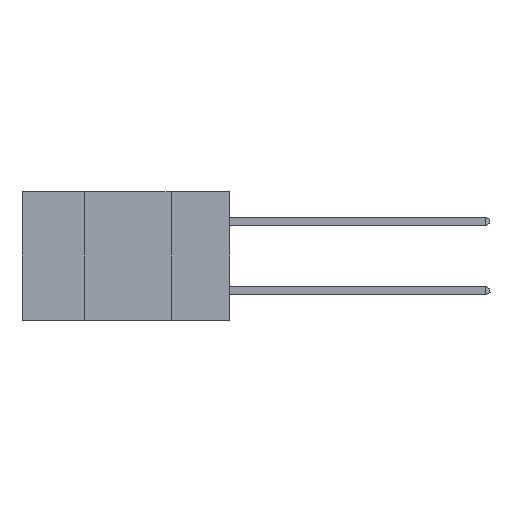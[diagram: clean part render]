
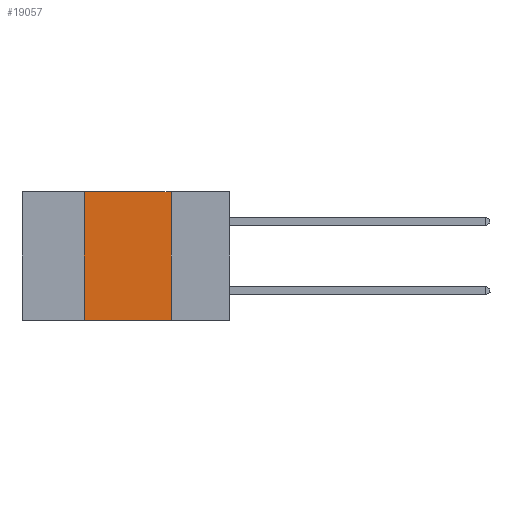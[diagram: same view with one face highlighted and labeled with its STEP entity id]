
A CAD part, left-side view. The second image highlights one B-rep face of the part: STEP entity #19057.
In plain terms, the highlighted planar face has unit normal (-1, 0, 0).
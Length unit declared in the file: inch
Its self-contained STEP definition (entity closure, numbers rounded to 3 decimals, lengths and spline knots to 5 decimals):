
#419 = CARTESIAN_POINT ( 'NONE',  ( 0., 0.17, 0. ) ) ;
#975 = FACE_OUTER_BOUND ( 'NONE', #11754, .T. ) ;
#3410 = EDGE_CURVE ( 'NONE', #18629, #6606, #17385, .T. ) ;
#5823 = VECTOR ( 'NONE', #15433, 39.37008 ) ;
#6005 = CARTESIAN_POINT ( 'NONE',  ( 0., 0.17, 0. ) ) ;
#6018 = PLANE ( 'NONE',  #11530 ) ;
#6328 = VERTEX_POINT ( 'NONE', #6005 ) ;
#6606 = VERTEX_POINT ( 'NONE', #8525 ) ;
#6717 = CARTESIAN_POINT ( 'NONE',  ( 0., 0.42, -0.37 ) ) ;
#6910 = DIRECTION ( 'NONE',  ( 0., 0., -1. ) ) ;
#7424 = ORIENTED_EDGE ( 'NONE', *, *, #16034, .F. ) ;
#8299 = DIRECTION ( 'NONE',  ( 1., 0., 0. ) ) ;
#8525 = CARTESIAN_POINT ( 'NONE',  ( 0., 0.42, 0. ) ) ;
#8859 = CARTESIAN_POINT ( 'NONE',  ( 0., 0.17, -0.37 ) ) ;
#9289 = LINE ( 'NONE', #419, #17434 ) ;
#9847 = CARTESIAN_POINT ( 'NONE',  ( 0., 0.6, -0.37 ) ) ;
#11530 = AXIS2_PLACEMENT_3D ( 'NONE', #21264, #8299, #25635 ) ;
#11754 = EDGE_LOOP ( 'NONE', ( #7424, #23258, #14090, #14635 ) ) ;
#14090 = ORIENTED_EDGE ( 'NONE', *, *, #3410, .F. ) ;
#14284 = CARTESIAN_POINT ( 'NONE',  ( 0., 0.6, 0. ) ) ;
#14635 = ORIENTED_EDGE ( 'NONE', *, *, #16087, .T. ) ;
#15156 = VERTEX_POINT ( 'NONE', #8859 ) ;
#15433 = DIRECTION ( 'NONE',  ( 0., 0., 1. ) ) ;
#16034 = EDGE_CURVE ( 'NONE', #6328, #15156, #9289, .T. ) ;
#16087 = EDGE_CURVE ( 'NONE', #18629, #15156, #20528, .T. ) ;
#17245 = CARTESIAN_POINT ( 'NONE',  ( 0., 0.42, 0. ) ) ;
#17385 = LINE ( 'NONE', #17245, #5823 ) ;
#17434 = VECTOR ( 'NONE', #6910, 39.37008 ) ;
#18629 = VERTEX_POINT ( 'NONE', #6717 ) ;
#19057 = ADVANCED_FACE ( 'NONE', ( #975 ), #6018, .F. ) ;
#19137 = VECTOR ( 'NONE', #24828, 39.37008 ) ;
#20528 = LINE ( 'NONE', #9847, #19137 ) ;
#21055 = EDGE_CURVE ( 'NONE', #6606, #6328, #22980, .T. ) ;
#21264 = CARTESIAN_POINT ( 'NONE',  ( 0., 0.6, 0. ) ) ;
#22980 = LINE ( 'NONE', #14284, #25038 ) ;
#23258 = ORIENTED_EDGE ( 'NONE', *, *, #21055, .F. ) ;
#24828 = DIRECTION ( 'NONE',  ( 0., -1., 0. ) ) ;
#25038 = VECTOR ( 'NONE', #27242, 39.37008 ) ;
#25635 = DIRECTION ( 'NONE',  ( 0., 0., -1. ) ) ;
#27242 = DIRECTION ( 'NONE',  ( 0., -1., 0. ) ) ;
